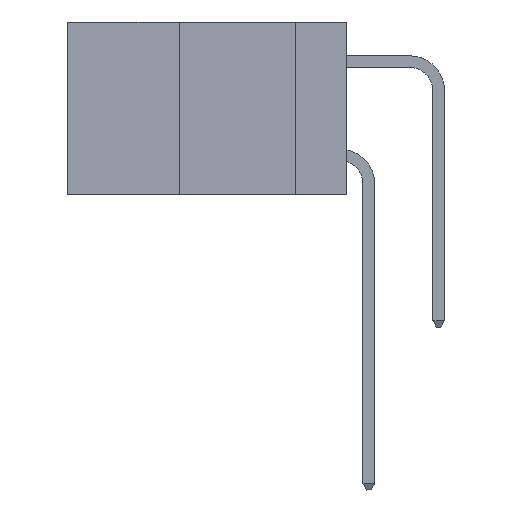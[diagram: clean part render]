
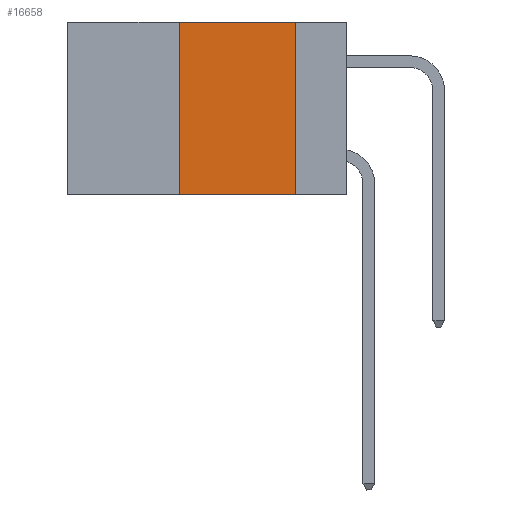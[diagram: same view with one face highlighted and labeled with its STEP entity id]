
A CAD part, left-side view. The second image highlights one B-rep face of the part: STEP entity #16658.
In plain terms, the highlighted planar face has unit normal (-1, 0, 0).
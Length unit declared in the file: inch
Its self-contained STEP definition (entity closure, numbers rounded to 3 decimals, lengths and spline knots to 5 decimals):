
#822 = DIRECTION ( 'NONE',  ( 0., 0., -1. ) ) ;
#1659 = LINE ( 'NONE', #20676, #20331 ) ;
#2938 = CARTESIAN_POINT ( 'NONE',  ( 0., 0.11, -0.37 ) ) ;
#3079 = DIRECTION ( 'NONE',  ( 0., 0., 1. ) ) ;
#3295 = LINE ( 'NONE', #7756, #23435 ) ;
#3492 = ORIENTED_EDGE ( 'NONE', *, *, #28290, .F. ) ;
#3734 = ORIENTED_EDGE ( 'NONE', *, *, #12991, .F. ) ;
#3997 = DIRECTION ( 'NONE',  ( 0., -1., 0. ) ) ;
#7756 = CARTESIAN_POINT ( 'NONE',  ( 0., 0.36, 0. ) ) ;
#8145 = VERTEX_POINT ( 'NONE', #20668 ) ;
#8189 = CARTESIAN_POINT ( 'NONE',  ( 0., 0.36, 0. ) ) ;
#10140 = CARTESIAN_POINT ( 'NONE',  ( 0., 0.36, -0.37 ) ) ;
#10981 = DIRECTION ( 'NONE',  ( 0., -1., 0. ) ) ;
#12749 = VERTEX_POINT ( 'NONE', #2938 ) ;
#12991 = EDGE_CURVE ( 'NONE', #8145, #12749, #14671, .T. ) ;
#13445 = DIRECTION ( 'NONE',  ( 1., 0., 0. ) ) ;
#14671 = LINE ( 'NONE', #18603, #19290 ) ;
#15235 = ORIENTED_EDGE ( 'NONE', *, *, #21656, .F. ) ;
#16658 = ADVANCED_FACE ( 'NONE', ( #17927 ), #27982, .F. ) ;
#17558 = LINE ( 'NONE', #28087, #19074 ) ;
#17927 = FACE_OUTER_BOUND ( 'NONE', #27299, .T. ) ;
#18390 = AXIS2_PLACEMENT_3D ( 'NONE', #29864, #13445, #822 ) ;
#18603 = CARTESIAN_POINT ( 'NONE',  ( 0., 0.11, 0. ) ) ;
#19074 = VECTOR ( 'NONE', #3997, 39.37008 ) ;
#19290 = VECTOR ( 'NONE', #30896, 39.37008 ) ;
#19481 = VERTEX_POINT ( 'NONE', #10140 ) ;
#20331 = VECTOR ( 'NONE', #10981, 39.37008 ) ;
#20668 = CARTESIAN_POINT ( 'NONE',  ( 0., 0.11, 0. ) ) ;
#20676 = CARTESIAN_POINT ( 'NONE',  ( 0., 0.6, -0.37 ) ) ;
#21656 = EDGE_CURVE ( 'NONE', #19481, #29311, #3295, .T. ) ;
#22576 = ORIENTED_EDGE ( 'NONE', *, *, #26580, .T. ) ;
#23435 = VECTOR ( 'NONE', #3079, 39.37008 ) ;
#26580 = EDGE_CURVE ( 'NONE', #19481, #12749, #1659, .T. ) ;
#27299 = EDGE_LOOP ( 'NONE', ( #3734, #3492, #15235, #22576 ) ) ;
#27982 = PLANE ( 'NONE',  #18390 ) ;
#28087 = CARTESIAN_POINT ( 'NONE',  ( 0., 0.6, 0. ) ) ;
#28290 = EDGE_CURVE ( 'NONE', #29311, #8145, #17558, .T. ) ;
#29311 = VERTEX_POINT ( 'NONE', #8189 ) ;
#29864 = CARTESIAN_POINT ( 'NONE',  ( 0., 0.6, 0. ) ) ;
#30896 = DIRECTION ( 'NONE',  ( 0., 0., -1. ) ) ;
